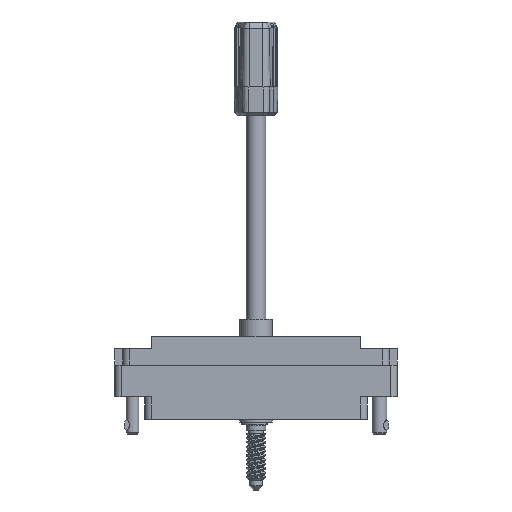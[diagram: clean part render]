
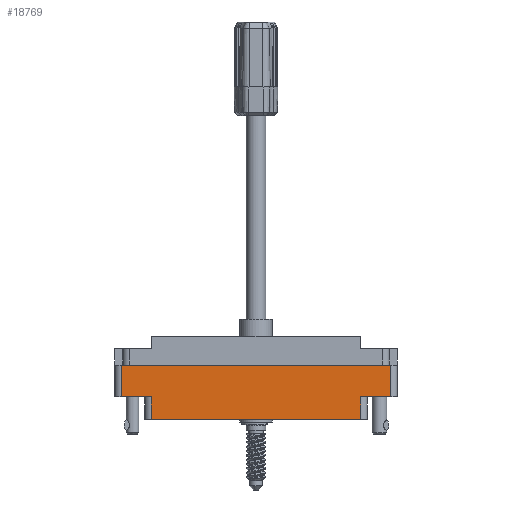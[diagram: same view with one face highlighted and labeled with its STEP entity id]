
A CAD part, front view. The second image highlights one B-rep face of the part: STEP entity #18769.
In plain terms, the highlighted planar face has unit normal (0, -1, 0).
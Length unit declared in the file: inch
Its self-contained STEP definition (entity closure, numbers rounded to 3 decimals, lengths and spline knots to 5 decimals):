
#2128 = LINE ( 'NONE', #36151, #23706 ) ;
#2993 = LINE ( 'NONE', #21861, #5175 ) ;
#5175 = VECTOR ( 'NONE', #14623, 39.37008 ) ;
#5983 = DIRECTION ( 'NONE',  ( 1., 0., 0. ) ) ;
#10639 = VERTEX_POINT ( 'NONE', #12379 ) ;
#10676 = ORIENTED_EDGE ( 'NONE', *, *, #60271, .T. ) ;
#11940 = LINE ( 'NONE', #40200, #82775 ) ;
#12379 = CARTESIAN_POINT ( 'NONE',  ( 1.006, -0.617, -0.798 ) ) ;
#14510 = EDGE_CURVE ( 'NONE', #10639, #85157, #16242, .T. ) ;
#14524 = CARTESIAN_POINT ( 'NONE',  ( -1.297, -0.617, -0.798 ) ) ;
#14623 = DIRECTION ( 'NONE',  ( 1., 0., 0. ) ) ;
#14827 = DIRECTION ( 'NONE',  ( 0., 0., -1. ) ) ;
#15206 = VECTOR ( 'NONE', #88735, 39.37008 ) ;
#16242 = LINE ( 'NONE', #84026, #22722 ) ;
#16501 = VERTEX_POINT ( 'NONE', #51823 ) ;
#16642 = EDGE_CURVE ( 'NONE', #17630, #33068, #2993, .T. ) ;
#17630 = VERTEX_POINT ( 'NONE', #20281 ) ;
#18769 = ADVANCED_FACE ( 'NONE', ( #59999 ), #80575, .T. ) ;
#19571 = LINE ( 'NONE', #60393, #41057 ) ;
#20281 = CARTESIAN_POINT ( 'NONE',  ( -1.297, -0.617, -0.274 ) ) ;
#21508 = EDGE_CURVE ( 'NONE', #77287, #62212, #51359, .T. ) ;
#21861 = CARTESIAN_POINT ( 'NONE',  ( 0., -0.617, -0.274 ) ) ;
#21881 = CARTESIAN_POINT ( 'NONE',  ( 1.297, -0.617, -0.274 ) ) ;
#22722 = VECTOR ( 'NONE', #85228, 39.37008 ) ;
#23706 = VECTOR ( 'NONE', #58981, 39.37008 ) ;
#24737 = ORIENTED_EDGE ( 'NONE', *, *, #34404, .T. ) ;
#24826 = DIRECTION ( 'NONE',  ( 0., -1., 0. ) ) ;
#28442 = CARTESIAN_POINT ( 'NONE',  ( -1.006, -0.617, -0.578 ) ) ;
#28824 = ORIENTED_EDGE ( 'NONE', *, *, #29751, .T. ) ;
#29004 = ORIENTED_EDGE ( 'NONE', *, *, #16642, .F. ) ;
#29751 = EDGE_CURVE ( 'NONE', #62212, #51596, #11940, .T. ) ;
#30296 = ORIENTED_EDGE ( 'NONE', *, *, #21508, .T. ) ;
#33068 = VERTEX_POINT ( 'NONE', #21881 ) ;
#34404 = EDGE_CURVE ( 'NONE', #51596, #10639, #19571, .T. ) ;
#35970 = LINE ( 'NONE', #14524, #83126 ) ;
#36151 = CARTESIAN_POINT ( 'NONE',  ( 1.297, -0.617, -0.798 ) ) ;
#38486 = VECTOR ( 'NONE', #62415, 39.37008 ) ;
#40200 = CARTESIAN_POINT ( 'NONE',  ( -1.006, -0.617, -0.798 ) ) ;
#40214 = CARTESIAN_POINT ( 'NONE',  ( -1.297, -0.617, -0.578 ) ) ;
#41057 = VECTOR ( 'NONE', #5983, 39.37008 ) ;
#41214 = CARTESIAN_POINT ( 'NONE',  ( 1.006, -0.617, -0.578 ) ) ;
#43371 = ORIENTED_EDGE ( 'NONE', *, *, #62946, .T. ) ;
#48357 = CARTESIAN_POINT ( 'NONE',  ( 0., -0.617, -0.578 ) ) ;
#51359 = LINE ( 'NONE', #48357, #38486 ) ;
#51596 = VERTEX_POINT ( 'NONE', #65391 ) ;
#51823 = CARTESIAN_POINT ( 'NONE',  ( 1.297, -0.617, -0.578 ) ) ;
#51854 = DIRECTION ( 'NONE',  ( 0., 0., -1. ) ) ;
#58981 = DIRECTION ( 'NONE',  ( 0., 0., 1. ) ) ;
#59999 = FACE_OUTER_BOUND ( 'NONE', #70526, .T. ) ;
#60271 = EDGE_CURVE ( 'NONE', #17630, #77287, #35970, .T. ) ;
#60393 = CARTESIAN_POINT ( 'NONE',  ( -1.359, -0.617, -0.798 ) ) ;
#62212 = VERTEX_POINT ( 'NONE', #28442 ) ;
#62415 = DIRECTION ( 'NONE',  ( 1., 0., 0. ) ) ;
#62946 = EDGE_CURVE ( 'NONE', #16501, #33068, #2128, .T. ) ;
#65391 = CARTESIAN_POINT ( 'NONE',  ( -1.006, -0.617, -0.798 ) ) ;
#65928 = CARTESIAN_POINT ( 'NONE',  ( -1.359, -0.617, -0.798 ) ) ;
#66253 = ORIENTED_EDGE ( 'NONE', *, *, #75531, .F. ) ;
#68037 = DIRECTION ( 'NONE',  ( 0., 0., -1. ) ) ;
#70003 = LINE ( 'NONE', #74935, #15206 ) ;
#70526 = EDGE_LOOP ( 'NONE', ( #30296, #28824, #24737, #80677, #66253, #43371, #29004, #10676 ) ) ;
#72175 = AXIS2_PLACEMENT_3D ( 'NONE', #65928, #24826, #51854 ) ;
#74935 = CARTESIAN_POINT ( 'NONE',  ( 0., -0.617, -0.578 ) ) ;
#75531 = EDGE_CURVE ( 'NONE', #16501, #85157, #70003, .T. ) ;
#77287 = VERTEX_POINT ( 'NONE', #40214 ) ;
#80575 = PLANE ( 'NONE',  #72175 ) ;
#80677 = ORIENTED_EDGE ( 'NONE', *, *, #14510, .T. ) ;
#82775 = VECTOR ( 'NONE', #68037, 39.37008 ) ;
#83126 = VECTOR ( 'NONE', #14827, 39.37008 ) ;
#84026 = CARTESIAN_POINT ( 'NONE',  ( 1.006, -0.617, -0.578 ) ) ;
#85157 = VERTEX_POINT ( 'NONE', #41214 ) ;
#85228 = DIRECTION ( 'NONE',  ( 0., 0., 1. ) ) ;
#88735 = DIRECTION ( 'NONE',  ( -1., 0., 0. ) ) ;
